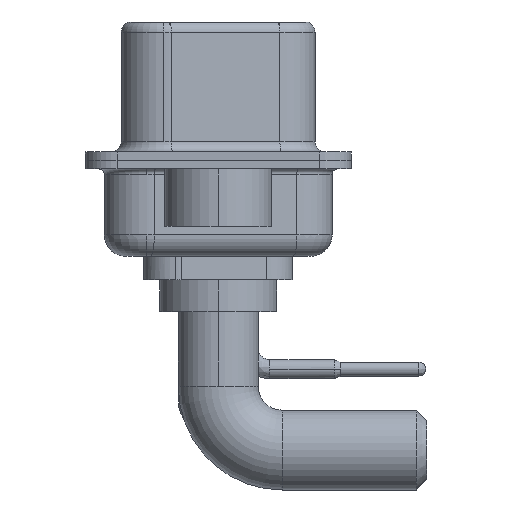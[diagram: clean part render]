
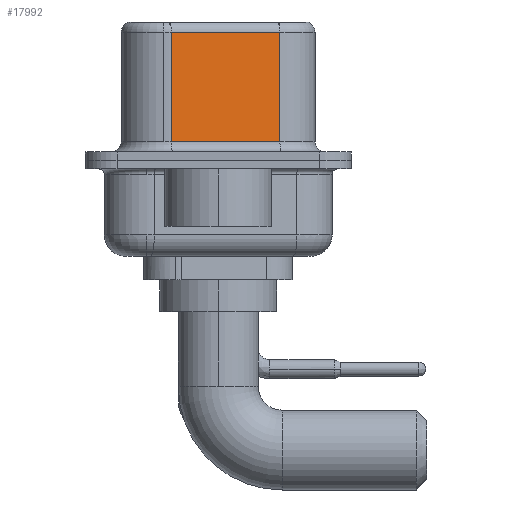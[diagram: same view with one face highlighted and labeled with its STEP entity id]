
A CAD part, left-side view. The second image highlights one B-rep face of the part: STEP entity #17992.
In plain terms, the highlighted planar face has unit normal (-0.985, -0.174, 0).
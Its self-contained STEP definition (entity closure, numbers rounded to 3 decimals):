
#88 = ORIENTED_EDGE ( 'NONE', *, *, #23428, .F. ) ;
#509 = DIRECTION ( 'NONE',  ( 0., 0., -1. ) ) ;
#653 = CARTESIAN_POINT ( 'NONE',  ( 4.58, -2.897, 6.52 ) ) ;
#819 = EDGE_LOOP ( 'NONE', ( #88, #23351, #23711, #17488 ) ) ;
#2069 = VECTOR ( 'NONE', #24924, 1000. ) ;
#2968 = CARTESIAN_POINT ( 'NONE',  ( 4.58, -2.897, 0.9 ) ) ;
#3529 = PLANE ( 'NONE',  #27791 ) ;
#4886 = VERTEX_POINT ( 'NONE', #20658 ) ;
#5216 = VECTOR ( 'NONE', #8408, 1000. ) ;
#6947 = CARTESIAN_POINT ( 'NONE',  ( 3.68, 2.203, 6.52 ) ) ;
#8403 = CARTESIAN_POINT ( 'NONE',  ( 4.58, -2.897, 6.52 ) ) ;
#8408 = DIRECTION ( 'NONE',  ( -0.174, 0.985, 0. ) ) ;
#9468 = EDGE_CURVE ( 'NONE', #26517, #21138, #24300, .T. ) ;
#9485 = CARTESIAN_POINT ( 'NONE',  ( 4.58, -2.897, 0.9 ) ) ;
#11652 = CARTESIAN_POINT ( 'NONE',  ( 3.68, 2.203, 6.02 ) ) ;
#12727 = VERTEX_POINT ( 'NONE', #2968 ) ;
#13028 = FACE_OUTER_BOUND ( 'NONE', #819, .T. ) ;
#13420 = EDGE_CURVE ( 'NONE', #4886, #26517, #19967, .T. ) ;
#15050 = CARTESIAN_POINT ( 'NONE',  ( 4.58, -2.897, 6.02 ) ) ;
#15756 = DIRECTION ( 'NONE',  ( 0., 0., -1. ) ) ;
#16629 = VECTOR ( 'NONE', #15756, 1000. ) ;
#17488 = ORIENTED_EDGE ( 'NONE', *, *, #27908, .T. ) ;
#17496 = DIRECTION ( 'NONE',  ( 0.985, 0.174, 0. ) ) ;
#17992 = ADVANCED_FACE ( 'NONE', ( #13028 ), #3529, .F. ) ;
#19967 = LINE ( 'NONE', #15050, #5216 ) ;
#20658 = CARTESIAN_POINT ( 'NONE',  ( 4.58, -2.897, 6.02 ) ) ;
#21001 = VECTOR ( 'NONE', #509, 1000. ) ;
#21138 = VERTEX_POINT ( 'NONE', #23996 ) ;
#21839 = DIRECTION ( 'NONE',  ( -0.174, 0.985, 0. ) ) ;
#23351 = ORIENTED_EDGE ( 'NONE', *, *, #13420, .T. ) ;
#23428 = EDGE_CURVE ( 'NONE', #4886, #12727, #24511, .T. ) ;
#23711 = ORIENTED_EDGE ( 'NONE', *, *, #9468, .T. ) ;
#23996 = CARTESIAN_POINT ( 'NONE',  ( 3.68, 2.203, 0.9 ) ) ;
#24300 = LINE ( 'NONE', #6947, #16629 ) ;
#24511 = LINE ( 'NONE', #653, #21001 ) ;
#24924 = DIRECTION ( 'NONE',  ( 0.174, -0.985, 0. ) ) ;
#26517 = VERTEX_POINT ( 'NONE', #11652 ) ;
#27521 = LINE ( 'NONE', #9485, #2069 ) ;
#27791 = AXIS2_PLACEMENT_3D ( 'NONE', #8403, #17496, #21839 ) ;
#27908 = EDGE_CURVE ( 'NONE', #21138, #12727, #27521, .T. ) ;
